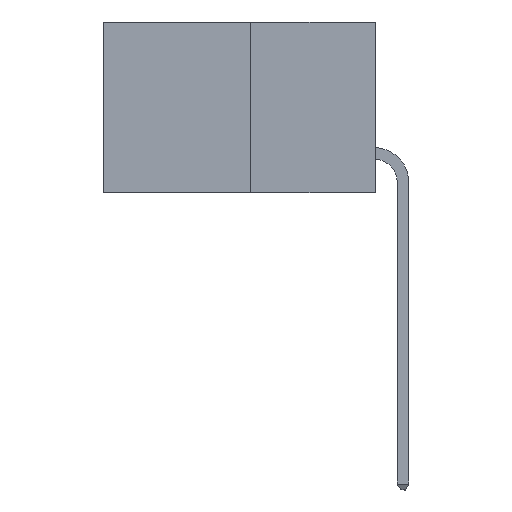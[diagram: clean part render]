
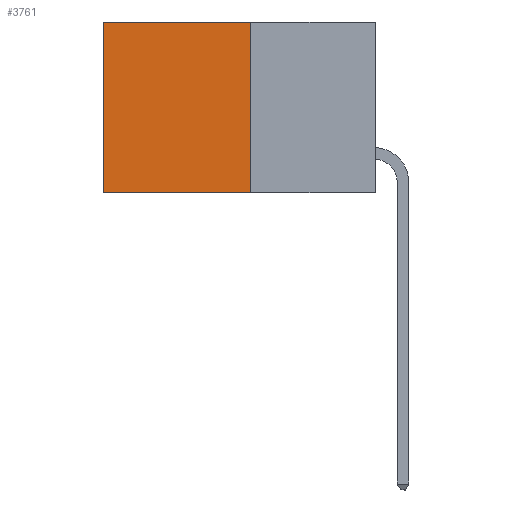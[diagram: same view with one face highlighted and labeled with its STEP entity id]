
A CAD part, left-side view. The second image highlights one B-rep face of the part: STEP entity #3761.
In plain terms, the highlighted planar face has unit normal (-1, 0, 0).
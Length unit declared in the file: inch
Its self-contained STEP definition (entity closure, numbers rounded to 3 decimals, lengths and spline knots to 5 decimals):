
#434 = DIRECTION ( 'NONE',  ( 1., 0., 0. ) ) ;
#445 = DIRECTION ( 'NONE',  ( 0., 0., -1. ) ) ;
#599 = ORIENTED_EDGE ( 'NONE', *, *, #1955, .F. ) ;
#694 = DIRECTION ( 'NONE',  ( 0., 0., -1. ) ) ;
#798 = PLANE ( 'NONE',  #5759 ) ;
#809 = CARTESIAN_POINT ( 'NONE',  ( 0.277, 0.27, -0.37 ) ) ;
#1217 = DIRECTION ( 'NONE',  ( 0., 0., -1. ) ) ;
#1665 = VERTEX_POINT ( 'NONE', #3415 ) ;
#1774 = VECTOR ( 'NONE', #10249, 39.37008 ) ;
#1955 = EDGE_CURVE ( 'NONE', #1665, #9087, #4412, .T. ) ;
#2502 = CARTESIAN_POINT ( 'NONE',  ( 0.277, 0.59, -0.37 ) ) ;
#3415 = CARTESIAN_POINT ( 'NONE',  ( 0.277, 0.27, -0.37 ) ) ;
#3761 = ADVANCED_FACE ( 'NONE', ( #5213 ), #798, .F. ) ;
#4202 = VECTOR ( 'NONE', #6862, 39.37008 ) ;
#4412 = LINE ( 'NONE', #8688, #1774 ) ;
#4530 = EDGE_LOOP ( 'NONE', ( #6645, #599, #7428, #10412 ) ) ;
#4703 = VERTEX_POINT ( 'NONE', #5637 ) ;
#4747 = CARTESIAN_POINT ( 'NONE',  ( 0.277, 0.27, -0.37 ) ) ;
#4983 = CARTESIAN_POINT ( 'NONE',  ( 0.277, 0.59, -0.37 ) ) ;
#5213 = FACE_OUTER_BOUND ( 'NONE', #4530, .T. ) ;
#5531 = CARTESIAN_POINT ( 'NONE',  ( 0.277, 0.27, 0. ) ) ;
#5637 = CARTESIAN_POINT ( 'NONE',  ( 0.277, 0.59, 0. ) ) ;
#5759 = AXIS2_PLACEMENT_3D ( 'NONE', #809, #434, #445 ) ;
#6259 = EDGE_CURVE ( 'NONE', #8841, #4703, #6521, .T. ) ;
#6521 = LINE ( 'NONE', #10962, #4202 ) ;
#6645 = ORIENTED_EDGE ( 'NONE', *, *, #9838, .T. ) ;
#6862 = DIRECTION ( 'NONE',  ( 0., 1., 0. ) ) ;
#7116 = VECTOR ( 'NONE', #1217, 39.37008 ) ;
#7428 = ORIENTED_EDGE ( 'NONE', *, *, #8924, .F. ) ;
#8260 = VECTOR ( 'NONE', #694, 39.37008 ) ;
#8688 = CARTESIAN_POINT ( 'NONE',  ( 0.277, 0.27, -0.37 ) ) ;
#8841 = VERTEX_POINT ( 'NONE', #5531 ) ;
#8924 = EDGE_CURVE ( 'NONE', #8841, #1665, #9560, .T. ) ;
#9087 = VERTEX_POINT ( 'NONE', #4983 ) ;
#9560 = LINE ( 'NONE', #4747, #7116 ) ;
#9838 = EDGE_CURVE ( 'NONE', #4703, #9087, #10461, .T. ) ;
#10249 = DIRECTION ( 'NONE',  ( 0., 1., 0. ) ) ;
#10412 = ORIENTED_EDGE ( 'NONE', *, *, #6259, .T. ) ;
#10461 = LINE ( 'NONE', #2502, #8260 ) ;
#10962 = CARTESIAN_POINT ( 'NONE',  ( 0.277, 0.27, 0. ) ) ;
